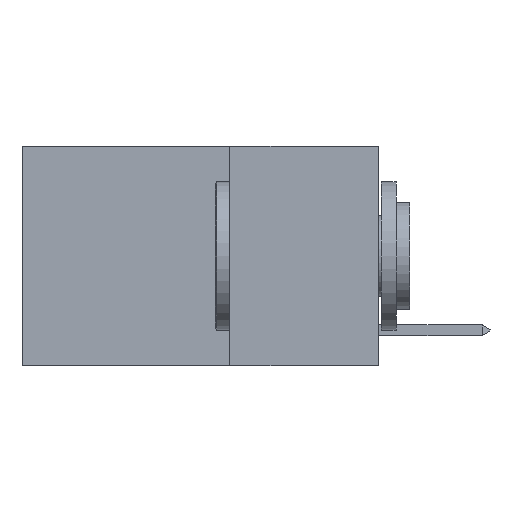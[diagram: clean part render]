
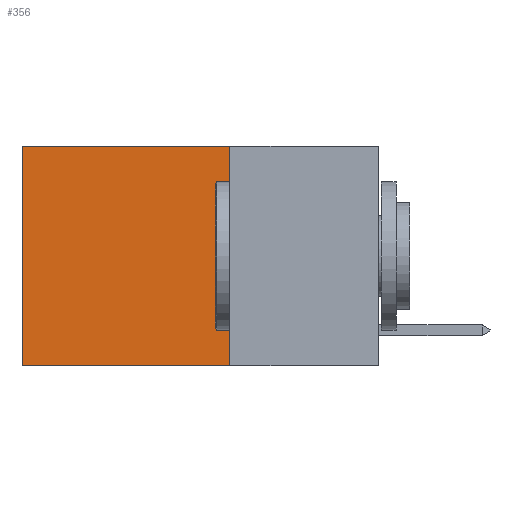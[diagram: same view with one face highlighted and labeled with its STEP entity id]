
A CAD part, left-side view. The second image highlights one B-rep face of the part: STEP entity #356.
In plain terms, the highlighted planar face has unit normal (-1, 0, 0).
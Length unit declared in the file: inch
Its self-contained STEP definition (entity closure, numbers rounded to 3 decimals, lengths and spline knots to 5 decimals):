
#356 = ADVANCED_FACE ( 'NONE', ( #8996 ), #5227, .F. ) ;
#470 = ORIENTED_EDGE ( 'NONE', *, *, #15671, .T. ) ;
#968 = VERTEX_POINT ( 'NONE', #15638 ) ;
#1620 = EDGE_CURVE ( 'NONE', #6663, #7081, #11210, .T. ) ;
#2028 = EDGE_LOOP ( 'NONE', ( #9846, #9519, #11522, #470 ) ) ;
#2385 = CARTESIAN_POINT ( 'NONE',  ( 0.2625, 0.25, -0.37 ) ) ;
#2481 = DIRECTION ( 'NONE',  ( 0., 1., 0. ) ) ;
#2900 = EDGE_CURVE ( 'NONE', #968, #7081, #13655, .T. ) ;
#3779 = AXIS2_PLACEMENT_3D ( 'NONE', #15260, #8917, #15498 ) ;
#4920 = DIRECTION ( 'NONE',  ( 0., 1., 0. ) ) ;
#5227 = PLANE ( 'NONE',  #3779 ) ;
#5820 = VECTOR ( 'NONE', #4920, 39.37008 ) ;
#6663 = VERTEX_POINT ( 'NONE', #2385 ) ;
#7000 = CARTESIAN_POINT ( 'NONE',  ( 0.2625, 0.6, 0. ) ) ;
#7081 = VERTEX_POINT ( 'NONE', #14640 ) ;
#7557 = VERTEX_POINT ( 'NONE', #16297 ) ;
#8917 = DIRECTION ( 'NONE',  ( 1., 0., 0. ) ) ;
#8996 = FACE_OUTER_BOUND ( 'NONE', #2028, .T. ) ;
#9009 = LINE ( 'NONE', #14157, #5820 ) ;
#9519 = ORIENTED_EDGE ( 'NONE', *, *, #1620, .F. ) ;
#9738 = EDGE_CURVE ( 'NONE', #7557, #6663, #13993, .T. ) ;
#9846 = ORIENTED_EDGE ( 'NONE', *, *, #2900, .T. ) ;
#11210 = LINE ( 'NONE', #14226, #14397 ) ;
#11260 = DIRECTION ( 'NONE',  ( 0., 0., -1. ) ) ;
#11522 = ORIENTED_EDGE ( 'NONE', *, *, #9738, .F. ) ;
#12561 = VECTOR ( 'NONE', #16288, 39.37008 ) ;
#13655 = LINE ( 'NONE', #7000, #12561 ) ;
#13993 = LINE ( 'NONE', #16444, #14868 ) ;
#14157 = CARTESIAN_POINT ( 'NONE',  ( 0.2625, 0.25, 0. ) ) ;
#14226 = CARTESIAN_POINT ( 'NONE',  ( 0.2625, 0.25, -0.37 ) ) ;
#14397 = VECTOR ( 'NONE', #2481, 39.37008 ) ;
#14640 = CARTESIAN_POINT ( 'NONE',  ( 0.2625, 0.6, -0.37 ) ) ;
#14868 = VECTOR ( 'NONE', #11260, 39.37008 ) ;
#15260 = CARTESIAN_POINT ( 'NONE',  ( 0.2625, 0.25, 0. ) ) ;
#15498 = DIRECTION ( 'NONE',  ( 0., 0., -1. ) ) ;
#15638 = CARTESIAN_POINT ( 'NONE',  ( 0.2625, 0.6, 0. ) ) ;
#15671 = EDGE_CURVE ( 'NONE', #7557, #968, #9009, .T. ) ;
#16288 = DIRECTION ( 'NONE',  ( 0., 0., -1. ) ) ;
#16297 = CARTESIAN_POINT ( 'NONE',  ( 0.2625, 0.25, 0. ) ) ;
#16444 = CARTESIAN_POINT ( 'NONE',  ( 0.2625, 0.25, 0. ) ) ;
